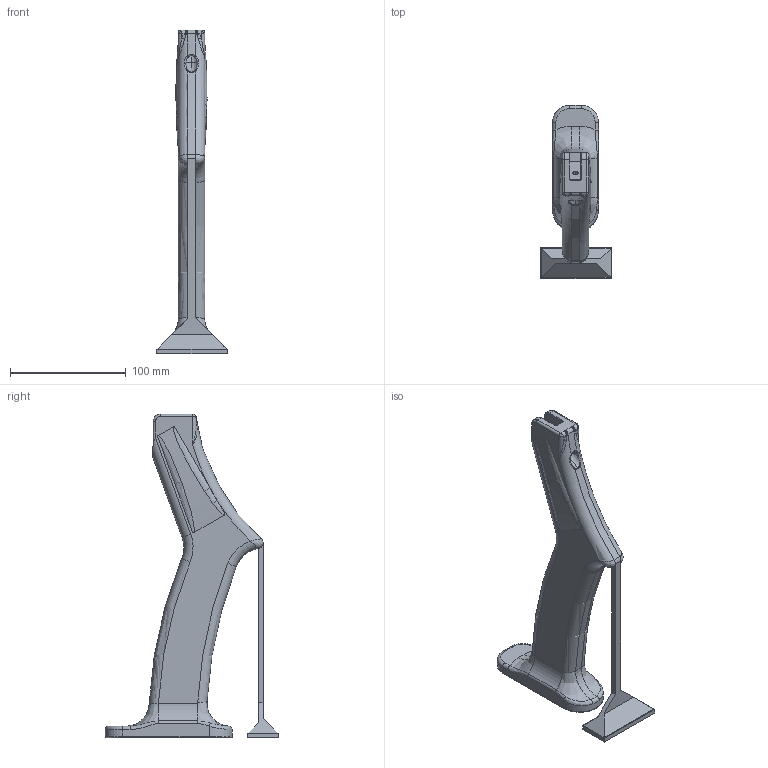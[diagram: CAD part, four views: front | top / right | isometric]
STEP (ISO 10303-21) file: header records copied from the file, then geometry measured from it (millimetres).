
FILE_DESCRIPTION((''),'2;1');
FILE_NAME('CMA','2014-02-13T',('Administrator'),(''),'PRO/ENGINEER BY PARAMETRIC TECHNOLOGY CORPORATION, 2012130','PRO/ENGINEER BY PARAMETRIC TECHNOLOGY CORPORATION, 2012130','');
FILE_SCHEMA(('CONFIG_CONTROL_DESIGN'));
Length unit declared in the file: millimetre
Products named in the file (1): CMA
Bounding box: 61.25 x 150.19 x 280 mm (x, y, z)
Volume: 302525.5 mm3; surface area: 72622.4 mm2
Topology: 1 solids, 3 shells, 206 faces, 485 edges, 286 vertices
Faces by surface type: cylinder 73, bspline 48, plane 47, torus 30, extrusion 4, sphere 4
Entity records: 9915 total; most frequent: CARTESIAN_POINT 5528, ORIENTED_EDGE 970, DIRECTION 825, EDGE_CURVE 485, AXIS2_PLACEMENT_3D 325, VERTEX_POINT 286, EDGE_LOOP 209, FACE_OUTER_BOUND 206
